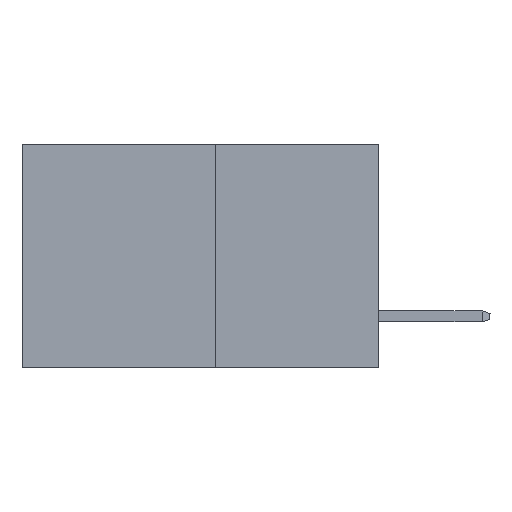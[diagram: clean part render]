
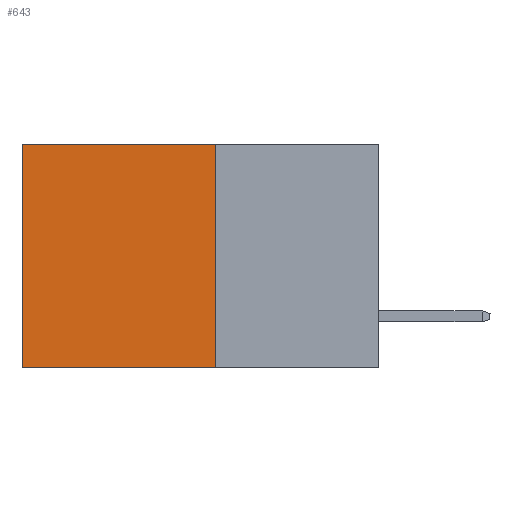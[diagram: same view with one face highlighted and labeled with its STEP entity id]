
A CAD part, left-side view. The second image highlights one B-rep face of the part: STEP entity #643.
In plain terms, the highlighted planar face has unit normal (-1, 0, 0).
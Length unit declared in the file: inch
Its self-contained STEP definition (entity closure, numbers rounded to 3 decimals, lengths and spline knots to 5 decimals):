
#13 = EDGE_CURVE ( 'NONE', #6502, #5986, #7021, .T. ) ;
#643 = ADVANCED_FACE ( 'NONE', ( #1181 ), #3568, .F. ) ;
#785 = CARTESIAN_POINT ( 'NONE',  ( 0.277, 0.27, 0. ) ) ;
#928 = DIRECTION ( 'NONE',  ( 0., 0., -1. ) ) ;
#1181 = FACE_OUTER_BOUND ( 'NONE', #7149, .T. ) ;
#2151 = CARTESIAN_POINT ( 'NONE',  ( 0.277, 0.59, -0.37 ) ) ;
#2188 = DIRECTION ( 'NONE',  ( 0., 0., -1. ) ) ;
#2285 = VERTEX_POINT ( 'NONE', #785 ) ;
#2314 = EDGE_CURVE ( 'NONE', #2285, #4989, #5640, .T. ) ;
#2362 = VECTOR ( 'NONE', #10310, 39.37008 ) ;
#3568 = PLANE ( 'NONE',  #10304 ) ;
#4141 = CARTESIAN_POINT ( 'NONE',  ( 0.277, 0.27, -0.37 ) ) ;
#4239 = CARTESIAN_POINT ( 'NONE',  ( 0.277, 0.27, 0. ) ) ;
#4470 = ORIENTED_EDGE ( 'NONE', *, *, #6901, .T. ) ;
#4508 = ORIENTED_EDGE ( 'NONE', *, *, #13, .F. ) ;
#4529 = ORIENTED_EDGE ( 'NONE', *, *, #9701, .F. ) ;
#4559 = ORIENTED_EDGE ( 'NONE', *, *, #2314, .T. ) ;
#4989 = VERTEX_POINT ( 'NONE', #6627 ) ;
#5107 = DIRECTION ( 'NONE',  ( 0., 1., 0. ) ) ;
#5184 = CARTESIAN_POINT ( 'NONE',  ( 0.277, 0.27, -0.37 ) ) ;
#5199 = CARTESIAN_POINT ( 'NONE',  ( 0.277, 0.27, -0.37 ) ) ;
#5260 = DIRECTION ( 'NONE',  ( 1., 0., 0. ) ) ;
#5366 = VECTOR ( 'NONE', #5107, 39.37008 ) ;
#5640 = LINE ( 'NONE', #4239, #5366 ) ;
#5986 = VERTEX_POINT ( 'NONE', #8605 ) ;
#6502 = VERTEX_POINT ( 'NONE', #5199 ) ;
#6627 = CARTESIAN_POINT ( 'NONE',  ( 0.277, 0.59, 0. ) ) ;
#6901 = EDGE_CURVE ( 'NONE', #4989, #5986, #9325, .T. ) ;
#6985 = CARTESIAN_POINT ( 'NONE',  ( 0.277, 0.27, -0.37 ) ) ;
#7021 = LINE ( 'NONE', #5184, #2362 ) ;
#7149 = EDGE_LOOP ( 'NONE', ( #4470, #4508, #4529, #4559 ) ) ;
#7995 = VECTOR ( 'NONE', #9987, 39.37008 ) ;
#8245 = LINE ( 'NONE', #4141, #7995 ) ;
#8605 = CARTESIAN_POINT ( 'NONE',  ( 0.277, 0.59, -0.37 ) ) ;
#9063 = VECTOR ( 'NONE', #2188, 39.37008 ) ;
#9325 = LINE ( 'NONE', #2151, #9063 ) ;
#9701 = EDGE_CURVE ( 'NONE', #2285, #6502, #8245, .T. ) ;
#9987 = DIRECTION ( 'NONE',  ( 0., 0., -1. ) ) ;
#10304 = AXIS2_PLACEMENT_3D ( 'NONE', #6985, #5260, #928 ) ;
#10310 = DIRECTION ( 'NONE',  ( 0., 1., 0. ) ) ;
